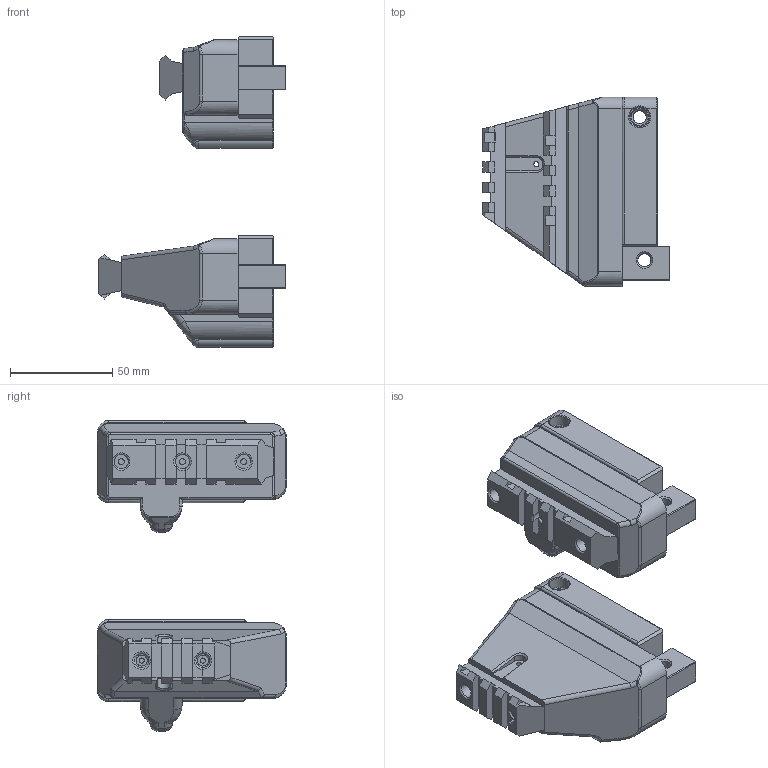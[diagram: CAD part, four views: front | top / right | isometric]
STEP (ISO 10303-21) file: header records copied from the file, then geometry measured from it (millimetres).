
FILE_DESCRIPTION(/* description */ (''),/* implementation_level */ '2;1');
FILE_NAME(/* name */ 'SIG brace rails and EC.stp',/* time_stamp */ '2021-05-19T23:08:48+02:00',/* author */ (''),/* organization */ (''),/* preprocessor_version */ 'ST-DEVELOPER v15.2',/* originating_system */ 'Autodesk Translator Framework v2.0.0.5431',/* authorisation */ '');
FILE_SCHEMA (('AUTOMOTIVE_DESIGN { 1 0 10303 214 3 1 1 }'));
Length unit declared in the file: centimetre
Products named in the file (1): (Unsaved)
Bounding box: 91.66 x 92.64 x 152.32 mm (x, y, z)
Volume: 309047.3 mm3; surface area: 66369.5 mm2
Topology: 4 solids, 4 shells, 556 faces, 1421 edges, 884 vertices
Faces by surface type: plane 297, cylinder 126, bspline 60, cone 41, torus 24, sphere 8
Full cylindrical faces by diameter (mm): 2.5 x6, 2.9 x6, 4 x2, 6.5 x6, 7 x5, 10 x4, 13 x2, 20.4 x1, 23.4 x2, 27.4 x2
Entity records: 19313 total; most frequent: CARTESIAN_POINT 6364, ORIENTED_EDGE 2668, DIRECTION 2556, EDGE_CURVE 1334, LINE 876, VECTOR 876, VERTEX_POINT 866, AXIS2_PLACEMENT_3D 840
